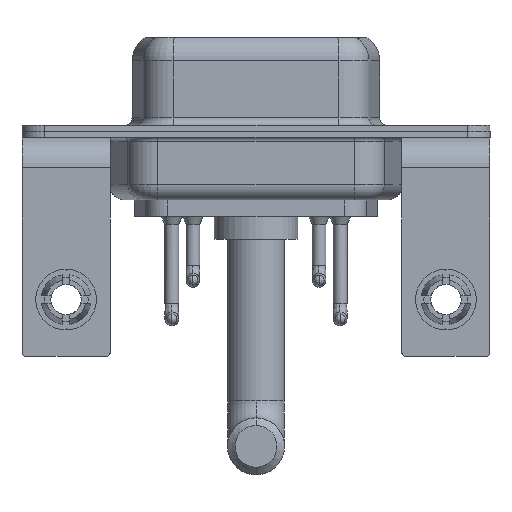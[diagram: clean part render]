
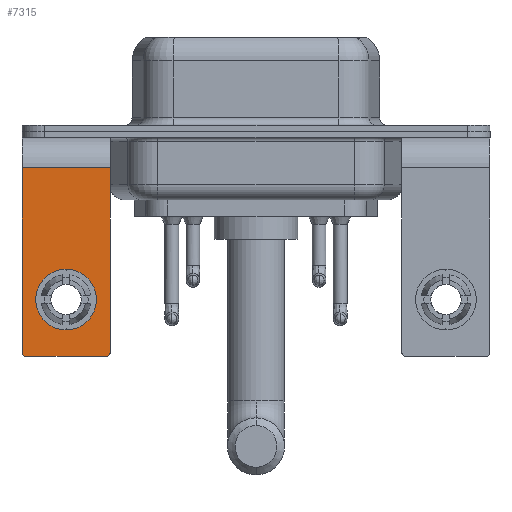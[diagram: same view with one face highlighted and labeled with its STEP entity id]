
A CAD part, front view. The second image highlights one B-rep face of the part: STEP entity #7315.
In plain terms, the highlighted planar face has unit normal (0, -1, 0).
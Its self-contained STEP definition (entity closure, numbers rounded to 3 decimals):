
#625 = CIRCLE ( 'NONE', #10897, 2. ) ;
#1072 = DIRECTION ( 'NONE',  ( 0., 1., 0. ) ) ;
#1137 = VERTEX_POINT ( 'NONE', #16659 ) ;
#1273 = VERTEX_POINT ( 'NONE', #12510 ) ;
#1327 = LINE ( 'NONE', #16939, #11437 ) ;
#1331 = CARTESIAN_POINT ( 'NONE',  ( 2.65, -6.25, -14.8 ) ) ;
#1407 = EDGE_CURVE ( 'NONE', #10076, #1137, #17129, .T. ) ;
#1470 = DIRECTION ( 'NONE',  ( 0., 1., 0. ) ) ;
#2246 = EDGE_CURVE ( 'NONE', #3188, #1273, #12550, .T. ) ;
#2382 = LINE ( 'NONE', #14131, #18674 ) ;
#2399 = FACE_OUTER_BOUND ( 'NONE', #16593, .T. ) ;
#2598 = CARTESIAN_POINT ( 'NONE',  ( -2.9, -6.25, -2.4 ) ) ;
#2671 = FACE_BOUND ( 'NONE', #12049, .T. ) ;
#3005 = VERTEX_POINT ( 'NONE', #9357 ) ;
#3188 = VERTEX_POINT ( 'NONE', #2598 ) ;
#3267 = AXIS2_PLACEMENT_3D ( 'NONE', #8644, #5781, #17587 ) ;
#3935 = VECTOR ( 'NONE', #4118, 1000. ) ;
#4072 = AXIS2_PLACEMENT_3D ( 'NONE', #13908, #7841, #13513 ) ;
#4118 = DIRECTION ( 'NONE',  ( -1., 0., 0. ) ) ;
#4380 = ORIENTED_EDGE ( 'NONE', *, *, #7786, .F. ) ;
#4728 = ORIENTED_EDGE ( 'NONE', *, *, #17355, .T. ) ;
#5308 = VERTEX_POINT ( 'NONE', #7685 ) ;
#5456 = DIRECTION ( 'NONE',  ( 0., 0., -1. ) ) ;
#5781 = DIRECTION ( 'NONE',  ( 0., -1., 0. ) ) ;
#5821 = ORIENTED_EDGE ( 'NONE', *, *, #9079, .T. ) ;
#6002 = CIRCLE ( 'NONE', #3267, 0.25 ) ;
#6141 = DIRECTION ( 'NONE',  ( 0., 1., 0. ) ) ;
#6598 = AXIS2_PLACEMENT_3D ( 'NONE', #16956, #1072, #18558 ) ;
#6935 = DIRECTION ( 'NONE',  ( -1., 0., 0. ) ) ;
#7130 = VECTOR ( 'NONE', #5456, 1000. ) ;
#7315 = ADVANCED_FACE ( 'NONE', ( #2671, #2399 ), #15571, .F. ) ;
#7562 = CARTESIAN_POINT ( 'NONE',  ( 0., -6.25, -11.07 ) ) ;
#7685 = CARTESIAN_POINT ( 'NONE',  ( 2.9, -6.25, -14.55 ) ) ;
#7786 = EDGE_CURVE ( 'NONE', #3005, #5308, #1327, .T. ) ;
#7790 = EDGE_CURVE ( 'NONE', #8999, #12412, #2382, .T. ) ;
#7841 = DIRECTION ( 'NONE',  ( 0., -1., 0. ) ) ;
#8644 = CARTESIAN_POINT ( 'NONE',  ( -2.65, -6.25, -14.55 ) ) ;
#8687 = CARTESIAN_POINT ( 'NONE',  ( 0., -6.25, -11.07 ) ) ;
#8999 = VERTEX_POINT ( 'NONE', #1331 ) ;
#9001 = DIRECTION ( 'NONE',  ( 0., 0., 1. ) ) ;
#9079 = EDGE_CURVE ( 'NONE', #1273, #12412, #6002, .T. ) ;
#9357 = CARTESIAN_POINT ( 'NONE',  ( 2.9, -6.25, -2.4 ) ) ;
#10076 = VERTEX_POINT ( 'NONE', #14712 ) ;
#10465 = ORIENTED_EDGE ( 'NONE', *, *, #1407, .T. ) ;
#10897 = AXIS2_PLACEMENT_3D ( 'NONE', #8687, #1470, #11684 ) ;
#11130 = LINE ( 'NONE', #18577, #3935 ) ;
#11437 = VECTOR ( 'NONE', #15464, 1000. ) ;
#11684 = DIRECTION ( 'NONE',  ( 0., 0., 1. ) ) ;
#12011 = CARTESIAN_POINT ( 'NONE',  ( -2.65, -6.25, -14.8 ) ) ;
#12049 = EDGE_LOOP ( 'NONE', ( #13940, #10465 ) ) ;
#12412 = VERTEX_POINT ( 'NONE', #12011 ) ;
#12510 = CARTESIAN_POINT ( 'NONE',  ( -2.9, -6.25, -14.55 ) ) ;
#12545 = CIRCLE ( 'NONE', #4072, 0.25 ) ;
#12550 = LINE ( 'NONE', #18303, #7130 ) ;
#13513 = DIRECTION ( 'NONE',  ( 0., 0., 1. ) ) ;
#13850 = AXIS2_PLACEMENT_3D ( 'NONE', #7562, #6141, #9001 ) ;
#13908 = CARTESIAN_POINT ( 'NONE',  ( 2.65, -6.25, -14.55 ) ) ;
#13940 = ORIENTED_EDGE ( 'NONE', *, *, #17693, .T. ) ;
#14131 = CARTESIAN_POINT ( 'NONE',  ( 2.9, -6.25, -14.8 ) ) ;
#14712 = CARTESIAN_POINT ( 'NONE',  ( 0., -6.25, -9.07 ) ) ;
#15317 = ORIENTED_EDGE ( 'NONE', *, *, #2246, .T. ) ;
#15464 = DIRECTION ( 'NONE',  ( 0., 0., -1. ) ) ;
#15571 = PLANE ( 'NONE',  #6598 ) ;
#16591 = ORIENTED_EDGE ( 'NONE', *, *, #7790, .F. ) ;
#16593 = EDGE_LOOP ( 'NONE', ( #15317, #5821, #16591, #4728, #4380, #18142 ) ) ;
#16659 = CARTESIAN_POINT ( 'NONE',  ( 0., -6.25, -13.07 ) ) ;
#16939 = CARTESIAN_POINT ( 'NONE',  ( 2.9, -6.25, -2.4 ) ) ;
#16956 = CARTESIAN_POINT ( 'NONE',  ( 2.9, -6.25, -2.4 ) ) ;
#17129 = CIRCLE ( 'NONE', #13850, 2. ) ;
#17355 = EDGE_CURVE ( 'NONE', #8999, #5308, #12545, .T. ) ;
#17473 = EDGE_CURVE ( 'NONE', #3005, #3188, #11130, .T. ) ;
#17587 = DIRECTION ( 'NONE',  ( 0., 0., 1. ) ) ;
#17693 = EDGE_CURVE ( 'NONE', #1137, #10076, #625, .T. ) ;
#18142 = ORIENTED_EDGE ( 'NONE', *, *, #17473, .T. ) ;
#18303 = CARTESIAN_POINT ( 'NONE',  ( -2.9, -6.25, -2.4 ) ) ;
#18558 = DIRECTION ( 'NONE',  ( 0., 0., 1. ) ) ;
#18577 = CARTESIAN_POINT ( 'NONE',  ( 2.9, -6.25, -2.4 ) ) ;
#18674 = VECTOR ( 'NONE', #6935, 1000. ) ;
